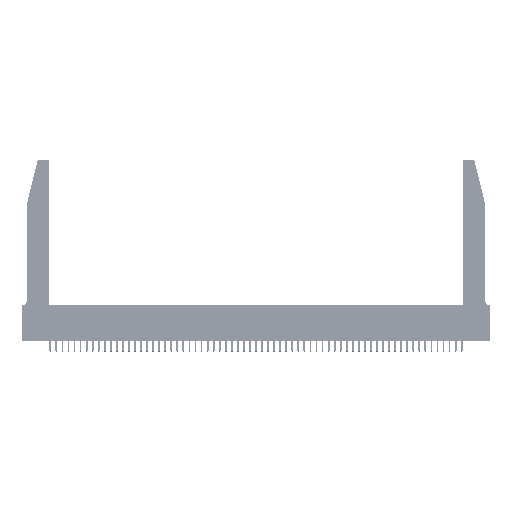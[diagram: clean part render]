
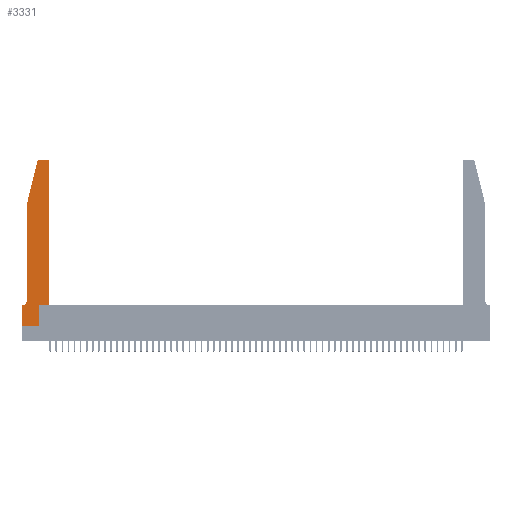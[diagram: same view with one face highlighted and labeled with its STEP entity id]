
A CAD part, top view. The second image highlights one B-rep face of the part: STEP entity #3331.
In plain terms, the highlighted planar face has unit normal (0, 0, 1).
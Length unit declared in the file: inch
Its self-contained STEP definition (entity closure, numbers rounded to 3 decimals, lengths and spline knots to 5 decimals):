
#475 = VERTEX_POINT ( 'NONE', #50444 ) ;
#814 = ORIENTED_EDGE ( 'NONE', *, *, #16043, .T. ) ;
#1594 = CARTESIAN_POINT ( 'NONE',  ( 0.284, 2.75, 0.37 ) ) ;
#1739 = CARTESIAN_POINT ( 'NONE',  ( 0.4505, 0.35, 0.37 ) ) ;
#2266 = EDGE_CURVE ( 'NONE', #49274, #7024, #15309, .T. ) ;
#3331 = ADVANCED_FACE ( 'NONE', ( #38894 ), #14965, .T. ) ;
#4902 = VERTEX_POINT ( 'NONE', #26087 ) ;
#5067 = ORIENTED_EDGE ( 'NONE', *, *, #2266, .T. ) ;
#5146 = ORIENTED_EDGE ( 'NONE', *, *, #9827, .T. ) ;
#6650 = LINE ( 'NONE', #43954, #19991 ) ;
#6766 = DIRECTION ( 'NONE',  ( 0., 0., 1. ) ) ;
#6857 = DIRECTION ( 'NONE',  ( -1., 0., 0. ) ) ;
#7024 = VERTEX_POINT ( 'NONE', #14260 ) ;
#7667 = VECTOR ( 'NONE', #16184, 39.37008 ) ;
#8536 = DIRECTION ( 'NONE',  ( 0., 0., 1. ) ) ;
#9827 = EDGE_CURVE ( 'NONE', #17948, #51659, #28120, .T. ) ;
#9961 = VECTOR ( 'NONE', #31652, 39.37008 ) ;
#10862 = EDGE_LOOP ( 'NONE', ( #55274, #29218, #20047, #43536, #11978, #814, #31862, #5067, #11561, #5146, #11433, #37193 ) ) ;
#11048 = VECTOR ( 'NONE', #37279, 39.37008 ) ;
#11131 = CARTESIAN_POINT ( 'NONE',  ( 0.0055, 0.35, 0.37 ) ) ;
#11433 = ORIENTED_EDGE ( 'NONE', *, *, #12920, .T. ) ;
#11561 = ORIENTED_EDGE ( 'NONE', *, *, #50330, .T. ) ;
#11912 = DIRECTION ( 'NONE',  ( 0., 1., 0. ) ) ;
#11978 = ORIENTED_EDGE ( 'NONE', *, *, #29759, .T. ) ;
#12099 = DIRECTION ( 'NONE',  ( 0., 0., -1. ) ) ;
#12259 = CARTESIAN_POINT ( 'NONE',  ( 0.4205, 2.72, 0.37 ) ) ;
#12305 = CIRCLE ( 'NONE', #17599, 0.07 ) ;
#12657 = VERTEX_POINT ( 'NONE', #54235 ) ;
#12920 = EDGE_CURVE ( 'NONE', #51659, #12657, #14594, .T. ) ;
#13297 = VERTEX_POINT ( 'NONE', #11131 ) ;
#13577 = AXIS2_PLACEMENT_3D ( 'NONE', #12259, #8536, #38484 ) ;
#14260 = CARTESIAN_POINT ( 'NONE',  ( 0.2865, 0., 0.37 ) ) ;
#14594 = LINE ( 'NONE', #1739, #9961 ) ;
#14669 = DIRECTION ( 'NONE',  ( 0., -1., 0. ) ) ;
#14965 = PLANE ( 'NONE',  #17926 ) ;
#15309 = LINE ( 'NONE', #33995, #28709 ) ;
#15620 = CARTESIAN_POINT ( 'NONE',  ( 0.0755, 0.35, 0.37 ) ) ;
#15695 = EDGE_CURVE ( 'NONE', #24027, #4902, #16392, .T. ) ;
#16043 = EDGE_CURVE ( 'NONE', #13297, #33677, #54570, .T. ) ;
#16184 = DIRECTION ( 'NONE',  ( -1., 0., 0. ) ) ;
#16201 = EDGE_CURVE ( 'NONE', #12657, #475, #27009, .T. ) ;
#16392 = LINE ( 'NONE', #28087, #11048 ) ;
#17148 = CARTESIAN_POINT ( 'NONE',  ( 0.25487, 2.72718, 0.37 ) ) ;
#17599 = AXIS2_PLACEMENT_3D ( 'NONE', #28766, #12099, #20512 ) ;
#17926 = AXIS2_PLACEMENT_3D ( 'NONE', #32412, #6766, #52607 ) ;
#17948 = VERTEX_POINT ( 'NONE', #18813 ) ;
#17993 = EDGE_CURVE ( 'NONE', #475, #32955, #25453, .T. ) ;
#18813 = CARTESIAN_POINT ( 'NONE',  ( 0.2865, 0.35, 0.37 ) ) ;
#19991 = VECTOR ( 'NONE', #26736, 39.37008 ) ;
#20047 = ORIENTED_EDGE ( 'NONE', *, *, #15695, .T. ) ;
#20512 = DIRECTION ( 'NONE',  ( -1., 0., 0. ) ) ;
#20732 = VECTOR ( 'NONE', #11912, 39.37008 ) ;
#21518 = CARTESIAN_POINT ( 'NONE',  ( 0.284, 2.72, 0.37 ) ) ;
#23570 = CARTESIAN_POINT ( 'NONE',  ( 0.4505, 0.35, 0.37 ) ) ;
#24027 = VERTEX_POINT ( 'NONE', #17148 ) ;
#25354 = DIRECTION ( 'NONE',  ( 1., 0., 0. ) ) ;
#25453 = LINE ( 'NONE', #28548, #32770 ) ;
#25742 = AXIS2_PLACEMENT_3D ( 'NONE', #21518, #38400, #29766 ) ;
#26087 = CARTESIAN_POINT ( 'NONE',  ( 0.0755, 2., 0.37 ) ) ;
#26292 = EDGE_CURVE ( 'NONE', #32955, #24027, #42940, .T. ) ;
#26736 = DIRECTION ( 'NONE',  ( 0., -1., 0. ) ) ;
#26760 = VECTOR ( 'NONE', #14669, 39.37008 ) ;
#27009 = CIRCLE ( 'NONE', #13577, 0.03 ) ;
#27867 = DIRECTION ( 'NONE',  ( 1., 0., 0. ) ) ;
#28087 = CARTESIAN_POINT ( 'NONE',  ( 0.0755, 2., 0.37 ) ) ;
#28120 = LINE ( 'NONE', #23570, #40830 ) ;
#28548 = CARTESIAN_POINT ( 'NONE',  ( 0.2605, 2.75, 0.37 ) ) ;
#28709 = VECTOR ( 'NONE', #25354, 39.37008 ) ;
#28766 = CARTESIAN_POINT ( 'NONE',  ( 0.0055, 0.42, 0.37 ) ) ;
#29218 = ORIENTED_EDGE ( 'NONE', *, *, #26292, .T. ) ;
#29759 = EDGE_CURVE ( 'NONE', #44185, #13297, #12305, .T. ) ;
#29766 = DIRECTION ( 'NONE',  ( 1., 0., 0. ) ) ;
#29897 = CARTESIAN_POINT ( 'NONE',  ( 0., 0., 0.37 ) ) ;
#30102 = LINE ( 'NONE', #40187, #26760 ) ;
#31652 = DIRECTION ( 'NONE',  ( 0., 1., 0. ) ) ;
#31862 = ORIENTED_EDGE ( 'NONE', *, *, #32292, .T. ) ;
#32292 = EDGE_CURVE ( 'NONE', #33677, #49274, #30102, .T. ) ;
#32412 = CARTESIAN_POINT ( 'NONE',  ( 0., 0.35, 0.37 ) ) ;
#32770 = VECTOR ( 'NONE', #6857, 39.37008 ) ;
#32955 = VERTEX_POINT ( 'NONE', #1594 ) ;
#33677 = VERTEX_POINT ( 'NONE', #48650 ) ;
#33995 = CARTESIAN_POINT ( 'NONE',  ( 0., 0., 0.37 ) ) ;
#37193 = ORIENTED_EDGE ( 'NONE', *, *, #16201, .T. ) ;
#37279 = DIRECTION ( 'NONE',  ( -0.239, -0.971, 0. ) ) ;
#38214 = EDGE_CURVE ( 'NONE', #4902, #44185, #6650, .T. ) ;
#38400 = DIRECTION ( 'NONE',  ( 0., 0., 1. ) ) ;
#38484 = DIRECTION ( 'NONE',  ( 1., 0., 0. ) ) ;
#38894 = FACE_OUTER_BOUND ( 'NONE', #10862, .T. ) ;
#40144 = CARTESIAN_POINT ( 'NONE',  ( 0.0755, 0.42, 0.37 ) ) ;
#40187 = CARTESIAN_POINT ( 'NONE',  ( 0., 0., 0.37 ) ) ;
#40203 = LINE ( 'NONE', #46528, #20732 ) ;
#40830 = VECTOR ( 'NONE', #27867, 39.37008 ) ;
#42664 = CARTESIAN_POINT ( 'NONE',  ( 0.4505, 0.35, 0.37 ) ) ;
#42940 = CIRCLE ( 'NONE', #25742, 0.03 ) ;
#43536 = ORIENTED_EDGE ( 'NONE', *, *, #38214, .T. ) ;
#43954 = CARTESIAN_POINT ( 'NONE',  ( 0.0755, 2., 0.37 ) ) ;
#44185 = VERTEX_POINT ( 'NONE', #40144 ) ;
#46528 = CARTESIAN_POINT ( 'NONE',  ( 0.2865, 0.35, 0.37 ) ) ;
#48650 = CARTESIAN_POINT ( 'NONE',  ( 0., 0.35, 0.37 ) ) ;
#49274 = VERTEX_POINT ( 'NONE', #29897 ) ;
#50330 = EDGE_CURVE ( 'NONE', #7024, #17948, #40203, .T. ) ;
#50444 = CARTESIAN_POINT ( 'NONE',  ( 0.4205, 2.75, 0.37 ) ) ;
#51659 = VERTEX_POINT ( 'NONE', #42664 ) ;
#52607 = DIRECTION ( 'NONE',  ( 1., 0., 0. ) ) ;
#54235 = CARTESIAN_POINT ( 'NONE',  ( 0.4505, 2.72, 0.37 ) ) ;
#54570 = LINE ( 'NONE', #15620, #7667 ) ;
#55274 = ORIENTED_EDGE ( 'NONE', *, *, #17993, .T. ) ;
